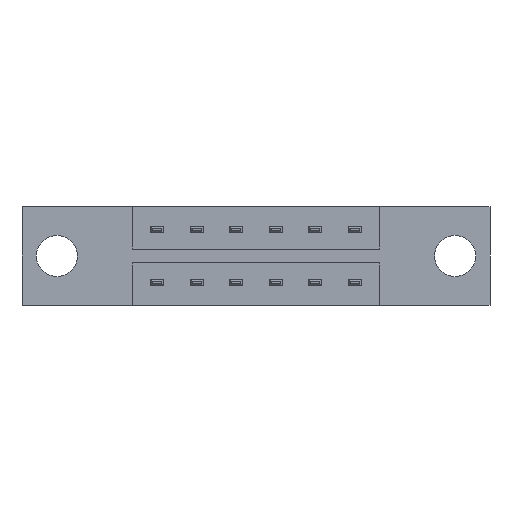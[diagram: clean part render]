
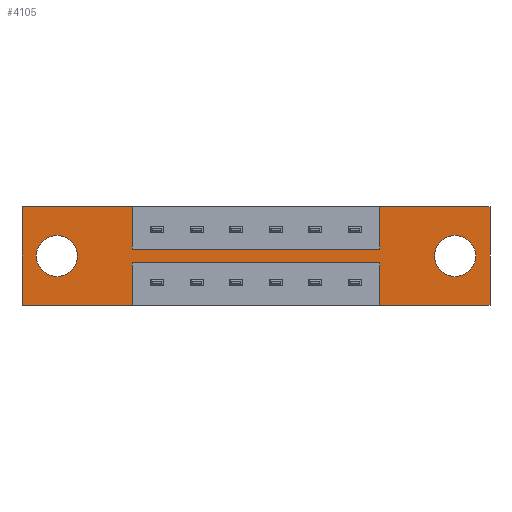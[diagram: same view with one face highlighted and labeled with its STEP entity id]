
A CAD part, front view. The second image highlights one B-rep face of the part: STEP entity #4105.
In plain terms, the highlighted planar face has unit normal (0, -1, 0).
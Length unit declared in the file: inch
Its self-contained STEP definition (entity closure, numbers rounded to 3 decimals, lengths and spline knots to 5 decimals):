
#60 = EDGE_CURVE ( 'NONE', #1665, #2411, #335, .T. ) ;
#84 = VECTOR ( 'NONE', #870, 39.37008 ) ;
#93 = LINE ( 'NONE', #4023, #501 ) ;
#98 = CARTESIAN_POINT ( 'NONE',  ( 1.6425, 0., -0.1875 ) ) ;
#131 = DIRECTION ( 'NONE',  ( 0., 0., -1. ) ) ;
#235 = VECTOR ( 'NONE', #560, 39.37008 ) ;
#256 = DIRECTION ( 'NONE',  ( 0., 1., 0. ) ) ;
#317 = DIRECTION ( 'NONE',  ( 0., 0., 1. ) ) ;
#335 = LINE ( 'NONE', #2806, #7689 ) ;
#339 = ORIENTED_EDGE ( 'NONE', *, *, #60, .F. ) ;
#342 = CARTESIAN_POINT ( 'NONE',  ( 0.1325, 0., -0.1875 ) ) ;
#374 = VERTEX_POINT ( 'NONE', #2441 ) ;
#451 = CARTESIAN_POINT ( 'NONE',  ( 0., 0., -0.375 ) ) ;
#501 = VECTOR ( 'NONE', #6938, 39.37008 ) ;
#529 = VECTOR ( 'NONE', #3765, 39.37008 ) ;
#560 = DIRECTION ( 'NONE',  ( 1., 0., 0. ) ) ;
#570 = VECTOR ( 'NONE', #6737, 39.37008 ) ;
#783 = VERTEX_POINT ( 'NONE', #6585 ) ;
#870 = DIRECTION ( 'NONE',  ( 1., 0., 0. ) ) ;
#961 = VECTOR ( 'NONE', #4511, 39.37008 ) ;
#1009 = CARTESIAN_POINT ( 'NONE',  ( 0.4175, 0., -0.161 ) ) ;
#1315 = CARTESIAN_POINT ( 'NONE',  ( 1.3575, 0., -0.375 ) ) ;
#1409 = DIRECTION ( 'NONE',  ( 0., 1., 0. ) ) ;
#1446 = EDGE_CURVE ( 'NONE', #3905, #3042, #2640, .T. ) ;
#1479 = EDGE_LOOP ( 'NONE', ( #7912, #3443, #6278, #4759, #4909, #3391, #7448, #4664, #7442, #2784, #3185, #339 ) ) ;
#1506 = CARTESIAN_POINT ( 'NONE',  ( 0.4175, 0., -0.214 ) ) ;
#1601 = LINE ( 'NONE', #451, #6534 ) ;
#1665 = VERTEX_POINT ( 'NONE', #6131 ) ;
#1672 = DIRECTION ( 'NONE',  ( 0., 0., 1. ) ) ;
#1674 = VECTOR ( 'NONE', #1672, 39.37008 ) ;
#1716 = LINE ( 'NONE', #5972, #6767 ) ;
#1829 = AXIS2_PLACEMENT_3D ( 'NONE', #6702, #2822, #7994 ) ;
#1852 = LINE ( 'NONE', #1009, #4678 ) ;
#1959 = EDGE_CURVE ( 'NONE', #3042, #8140, #1716, .T. ) ;
#2171 = CARTESIAN_POINT ( 'NONE',  ( 1.6425, 0., -0.1875 ) ) ;
#2192 = CARTESIAN_POINT ( 'NONE',  ( 0.4175, 0., -0.161 ) ) ;
#2250 = LINE ( 'NONE', #3147, #529 ) ;
#2278 = LINE ( 'NONE', #2192, #570 ) ;
#2342 = LINE ( 'NONE', #2552, #961 ) ;
#2411 = VERTEX_POINT ( 'NONE', #1506 ) ;
#2426 = EDGE_CURVE ( 'NONE', #7171, #1665, #93, .T. ) ;
#2441 = CARTESIAN_POINT ( 'NONE',  ( 0.1325, 0., -0.1095 ) ) ;
#2552 = CARTESIAN_POINT ( 'NONE',  ( 0.4175, 0., -0.214 ) ) ;
#2633 = CIRCLE ( 'NONE', #4803, 0.078 ) ;
#2640 = LINE ( 'NONE', #2918, #235 ) ;
#2645 = EDGE_CURVE ( 'NONE', #8064, #3206, #7158, .T. ) ;
#2725 = DIRECTION ( 'NONE',  ( 0., 0., -1. ) ) ;
#2748 = CIRCLE ( 'NONE', #4108, 0.078 ) ;
#2759 = EDGE_LOOP ( 'NONE', ( #3923, #5918 ) ) ;
#2764 = CARTESIAN_POINT ( 'NONE',  ( 1.775, 0., 0. ) ) ;
#2784 = ORIENTED_EDGE ( 'NONE', *, *, #5465, .F. ) ;
#2790 = EDGE_CURVE ( 'NONE', #8271, #374, #7549, .T. ) ;
#2806 = CARTESIAN_POINT ( 'NONE',  ( 0.4175, 0., -0.214 ) ) ;
#2809 = FACE_BOUND ( 'NONE', #4823, .T. ) ;
#2822 = DIRECTION ( 'NONE',  ( 0., -1., 0. ) ) ;
#2851 = DIRECTION ( 'NONE',  ( 0., 0., 1. ) ) ;
#2918 = CARTESIAN_POINT ( 'NONE',  ( 0., 0., 0. ) ) ;
#3042 = VERTEX_POINT ( 'NONE', #2764 ) ;
#3147 = CARTESIAN_POINT ( 'NONE',  ( 0., 0., 0. ) ) ;
#3185 = ORIENTED_EDGE ( 'NONE', *, *, #6671, .F. ) ;
#3206 = VERTEX_POINT ( 'NONE', #4548 ) ;
#3350 = CARTESIAN_POINT ( 'NONE',  ( 0.1325, 0., -0.1875 ) ) ;
#3391 = ORIENTED_EDGE ( 'NONE', *, *, #5224, .F. ) ;
#3443 = ORIENTED_EDGE ( 'NONE', *, *, #4295, .F. ) ;
#3632 = CARTESIAN_POINT ( 'NONE',  ( 0., 0., -0.375 ) ) ;
#3765 = DIRECTION ( 'NONE',  ( 0., 0., 1. ) ) ;
#3768 = CARTESIAN_POINT ( 'NONE',  ( 1.3575, 0., 0. ) ) ;
#3903 = CARTESIAN_POINT ( 'NONE',  ( 0.1325, 0., -0.2655 ) ) ;
#3905 = VERTEX_POINT ( 'NONE', #3768 ) ;
#3923 = ORIENTED_EDGE ( 'NONE', *, *, #7520, .T. ) ;
#3963 = ORIENTED_EDGE ( 'NONE', *, *, #2790, .T. ) ;
#4008 = DIRECTION ( 'NONE',  ( -1., 0., 0. ) ) ;
#4023 = CARTESIAN_POINT ( 'NONE',  ( 1.3575, 0., -0.214 ) ) ;
#4037 = AXIS2_PLACEMENT_3D ( 'NONE', #342, #4862, #317 ) ;
#4105 = ADVANCED_FACE ( 'NONE', ( #4903, #2809, #5706 ), #8018, .T. ) ;
#4108 = AXIS2_PLACEMENT_3D ( 'NONE', #3350, #4740, #2851 ) ;
#4268 = VERTEX_POINT ( 'NONE', #4864 ) ;
#4295 = EDGE_CURVE ( 'NONE', #8140, #7171, #1601, .T. ) ;
#4511 = DIRECTION ( 'NONE',  ( 0., 0., -1. ) ) ;
#4548 = CARTESIAN_POINT ( 'NONE',  ( 0.4175, 0., 0. ) ) ;
#4622 = VERTEX_POINT ( 'NONE', #4779 ) ;
#4664 = ORIENTED_EDGE ( 'NONE', *, *, #2645, .F. ) ;
#4678 = VECTOR ( 'NONE', #6186, 39.37008 ) ;
#4740 = DIRECTION ( 'NONE',  ( 0., 1., 0. ) ) ;
#4759 = ORIENTED_EDGE ( 'NONE', *, *, #1446, .F. ) ;
#4779 = CARTESIAN_POINT ( 'NONE',  ( 1.6425, 0., -0.2655 ) ) ;
#4803 = AXIS2_PLACEMENT_3D ( 'NONE', #2171, #256, #2725 ) ;
#4823 = EDGE_LOOP ( 'NONE', ( #4858, #3963 ) ) ;
#4858 = ORIENTED_EDGE ( 'NONE', *, *, #7313, .T. ) ;
#4862 = DIRECTION ( 'NONE',  ( 0., 1., 0. ) ) ;
#4864 = CARTESIAN_POINT ( 'NONE',  ( 0.4175, 0., -0.375 ) ) ;
#4903 = FACE_BOUND ( 'NONE', #2759, .T. ) ;
#4909 = ORIENTED_EDGE ( 'NONE', *, *, #7895, .F. ) ;
#5224 = EDGE_CURVE ( 'NONE', #7109, #783, #2278, .T. ) ;
#5465 = EDGE_CURVE ( 'NONE', #4268, #6654, #8325, .T. ) ;
#5628 = EDGE_CURVE ( 'NONE', #4622, #5993, #7221, .T. ) ;
#5706 = FACE_OUTER_BOUND ( 'NONE', #1479, .T. ) ;
#5710 = CARTESIAN_POINT ( 'NONE',  ( 0., 0., -0.375 ) ) ;
#5918 = ORIENTED_EDGE ( 'NONE', *, *, #5628, .T. ) ;
#5972 = CARTESIAN_POINT ( 'NONE',  ( 1.775, 0., 0. ) ) ;
#5993 = VERTEX_POINT ( 'NONE', #8245 ) ;
#5994 = LINE ( 'NONE', #6793, #1674 ) ;
#6131 = CARTESIAN_POINT ( 'NONE',  ( 1.3575, 0., -0.214 ) ) ;
#6186 = DIRECTION ( 'NONE',  ( 0., 0., -1. ) ) ;
#6278 = ORIENTED_EDGE ( 'NONE', *, *, #1959, .F. ) ;
#6534 = VECTOR ( 'NONE', #8062, 39.37008 ) ;
#6585 = CARTESIAN_POINT ( 'NONE',  ( 1.3575, 0., -0.161 ) ) ;
#6644 = CARTESIAN_POINT ( 'NONE',  ( 0., 0., 0. ) ) ;
#6654 = VERTEX_POINT ( 'NONE', #5710 ) ;
#6671 = EDGE_CURVE ( 'NONE', #2411, #4268, #2342, .T. ) ;
#6702 = CARTESIAN_POINT ( 'NONE',  ( 0., 0., -0.375 ) ) ;
#6737 = DIRECTION ( 'NONE',  ( 1., 0., 0. ) ) ;
#6767 = VECTOR ( 'NONE', #7885, 39.37008 ) ;
#6793 = CARTESIAN_POINT ( 'NONE',  ( 1.3575, 0., -0.161 ) ) ;
#6862 = EDGE_CURVE ( 'NONE', #3206, #7109, #1852, .T. ) ;
#6904 = CARTESIAN_POINT ( 'NONE',  ( 0., 0., 0. ) ) ;
#6921 = DIRECTION ( 'NONE',  ( -1., 0., 0. ) ) ;
#6938 = DIRECTION ( 'NONE',  ( 0., 0., 1. ) ) ;
#6983 = CARTESIAN_POINT ( 'NONE',  ( 1.775, 0., -0.375 ) ) ;
#7082 = CARTESIAN_POINT ( 'NONE',  ( 0.4175, 0., -0.161 ) ) ;
#7109 = VERTEX_POINT ( 'NONE', #7082 ) ;
#7158 = LINE ( 'NONE', #6644, #84 ) ;
#7171 = VERTEX_POINT ( 'NONE', #1315 ) ;
#7194 = EDGE_CURVE ( 'NONE', #6654, #8064, #2250, .T. ) ;
#7221 = CIRCLE ( 'NONE', #7953, 0.078 ) ;
#7231 = VECTOR ( 'NONE', #6921, 39.37008 ) ;
#7313 = EDGE_CURVE ( 'NONE', #374, #8271, #2748, .T. ) ;
#7442 = ORIENTED_EDGE ( 'NONE', *, *, #7194, .F. ) ;
#7448 = ORIENTED_EDGE ( 'NONE', *, *, #6862, .F. ) ;
#7520 = EDGE_CURVE ( 'NONE', #5993, #4622, #2633, .T. ) ;
#7549 = CIRCLE ( 'NONE', #4037, 0.078 ) ;
#7689 = VECTOR ( 'NONE', #4008, 39.37008 ) ;
#7885 = DIRECTION ( 'NONE',  ( 0., 0., -1. ) ) ;
#7895 = EDGE_CURVE ( 'NONE', #783, #3905, #5994, .T. ) ;
#7912 = ORIENTED_EDGE ( 'NONE', *, *, #2426, .F. ) ;
#7953 = AXIS2_PLACEMENT_3D ( 'NONE', #98, #1409, #131 ) ;
#7994 = DIRECTION ( 'NONE',  ( 0., 0., -1. ) ) ;
#8018 = PLANE ( 'NONE',  #1829 ) ;
#8062 = DIRECTION ( 'NONE',  ( -1., 0., 0. ) ) ;
#8064 = VERTEX_POINT ( 'NONE', #6904 ) ;
#8140 = VERTEX_POINT ( 'NONE', #6983 ) ;
#8245 = CARTESIAN_POINT ( 'NONE',  ( 1.6425, 0., -0.1095 ) ) ;
#8271 = VERTEX_POINT ( 'NONE', #3903 ) ;
#8325 = LINE ( 'NONE', #3632, #7231 ) ;
